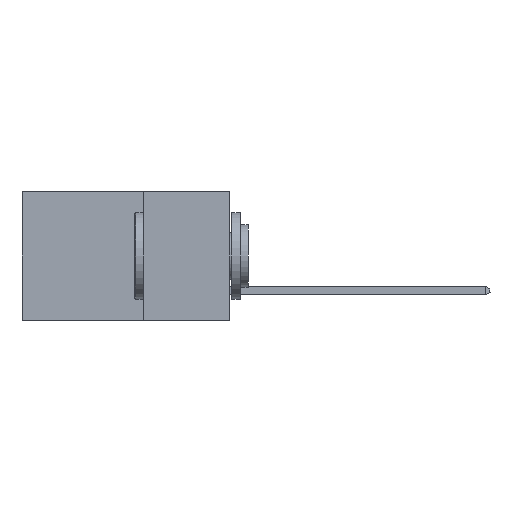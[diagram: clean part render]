
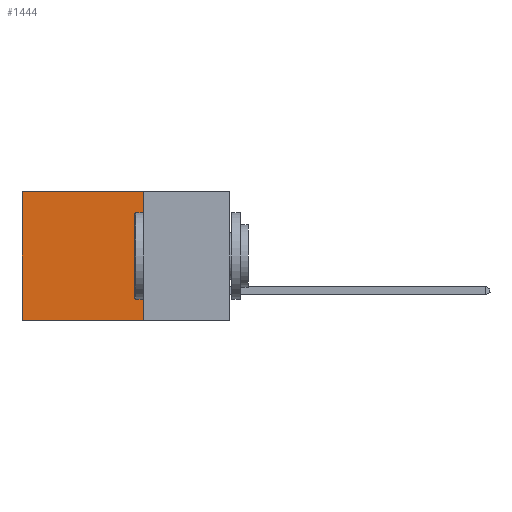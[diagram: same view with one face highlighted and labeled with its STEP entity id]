
A CAD part, left-side view. The second image highlights one B-rep face of the part: STEP entity #1444.
In plain terms, the highlighted planar face has unit normal (-1, 0, 0).
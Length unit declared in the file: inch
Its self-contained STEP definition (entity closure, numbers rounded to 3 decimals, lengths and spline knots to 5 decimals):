
#838 = VECTOR ( 'NONE', #1402, 39.37008 ) ;
#1357 = FACE_OUTER_BOUND ( 'NONE', #18709, .T. ) ;
#1402 = DIRECTION ( 'NONE',  ( 0., 0., -1. ) ) ;
#1444 = ADVANCED_FACE ( 'NONE', ( #1357 ), #6517, .F. ) ;
#1863 = CARTESIAN_POINT ( 'NONE',  ( 0.298, 0.6, 0. ) ) ;
#1975 = VECTOR ( 'NONE', #6210, 39.37008 ) ;
#2078 = CARTESIAN_POINT ( 'NONE',  ( 0.298, 0.25, 0. ) ) ;
#2175 = CARTESIAN_POINT ( 'NONE',  ( 0.298, 0.6, -0.37 ) ) ;
#2213 = LINE ( 'NONE', #1863, #838 ) ;
#2358 = EDGE_CURVE ( 'NONE', #11095, #17976, #2213, .T. ) ;
#2692 = VERTEX_POINT ( 'NONE', #13581 ) ;
#3623 = DIRECTION ( 'NONE',  ( 1., 0., 0. ) ) ;
#3824 = CARTESIAN_POINT ( 'NONE',  ( 0.298, 0.25, 0. ) ) ;
#4148 = DIRECTION ( 'NONE',  ( 0., 1., 0. ) ) ;
#4272 = LINE ( 'NONE', #14038, #7013 ) ;
#4761 = EDGE_CURVE ( 'NONE', #17510, #2692, #15254, .T. ) ;
#4785 = EDGE_CURVE ( 'NONE', #2692, #17976, #4272, .T. ) ;
#5702 = ORIENTED_EDGE ( 'NONE', *, *, #5988, .T. ) ;
#5925 = AXIS2_PLACEMENT_3D ( 'NONE', #3824, #3623, #16948 ) ;
#5988 = EDGE_CURVE ( 'NONE', #17510, #11095, #18192, .T. ) ;
#6210 = DIRECTION ( 'NONE',  ( 0., 0., -1. ) ) ;
#6517 = PLANE ( 'NONE',  #5925 ) ;
#7013 = VECTOR ( 'NONE', #15348, 39.37008 ) ;
#7239 = ORIENTED_EDGE ( 'NONE', *, *, #4785, .F. ) ;
#8700 = CARTESIAN_POINT ( 'NONE',  ( 0.298, 0.6, 0. ) ) ;
#8720 = CARTESIAN_POINT ( 'NONE',  ( 0.298, 0.25, 0. ) ) ;
#11095 = VERTEX_POINT ( 'NONE', #8700 ) ;
#13581 = CARTESIAN_POINT ( 'NONE',  ( 0.298, 0.25, -0.37 ) ) ;
#14038 = CARTESIAN_POINT ( 'NONE',  ( 0.298, 0.25, -0.37 ) ) ;
#15095 = ORIENTED_EDGE ( 'NONE', *, *, #4761, .F. ) ;
#15254 = LINE ( 'NONE', #17979, #1975 ) ;
#15348 = DIRECTION ( 'NONE',  ( 0., 1., 0. ) ) ;
#16948 = DIRECTION ( 'NONE',  ( 0., 0., -1. ) ) ;
#17269 = VECTOR ( 'NONE', #4148, 39.37008 ) ;
#17510 = VERTEX_POINT ( 'NONE', #2078 ) ;
#17976 = VERTEX_POINT ( 'NONE', #2175 ) ;
#17979 = CARTESIAN_POINT ( 'NONE',  ( 0.298, 0.25, 0. ) ) ;
#18188 = ORIENTED_EDGE ( 'NONE', *, *, #2358, .T. ) ;
#18192 = LINE ( 'NONE', #8720, #17269 ) ;
#18709 = EDGE_LOOP ( 'NONE', ( #18188, #7239, #15095, #5702 ) ) ;
